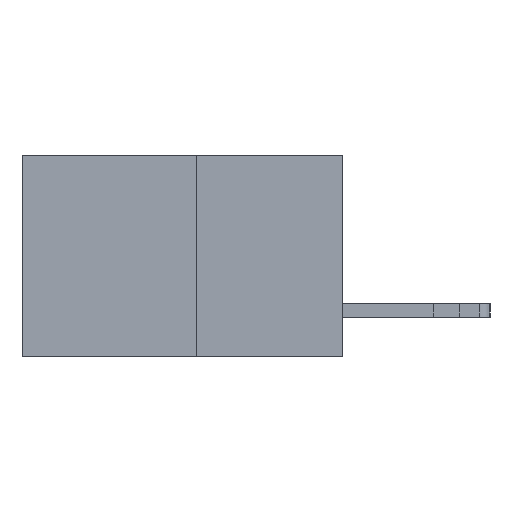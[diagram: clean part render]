
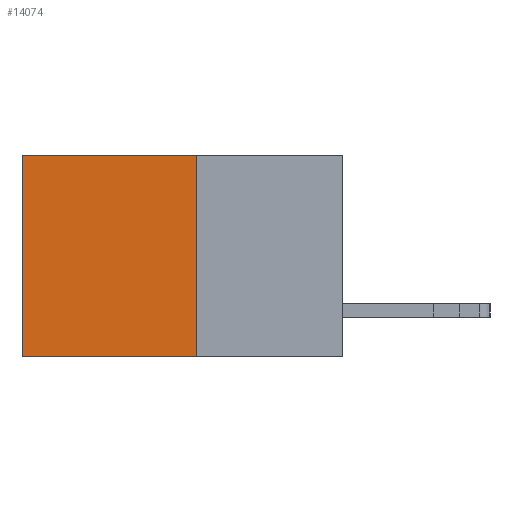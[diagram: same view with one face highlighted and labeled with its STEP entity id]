
A CAD part, left-side view. The second image highlights one B-rep face of the part: STEP entity #14074.
In plain terms, the highlighted planar face has unit normal (-1, 0, 0).
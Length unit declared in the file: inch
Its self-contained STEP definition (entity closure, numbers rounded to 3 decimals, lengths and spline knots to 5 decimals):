
#110 = CARTESIAN_POINT ( 'NONE',  ( 0.277, 0.27, -0.37 ) ) ;
#305 = EDGE_CURVE ( 'NONE', #2787, #11590, #13368, .T. ) ;
#1019 = DIRECTION ( 'NONE',  ( 0., 1., 0. ) ) ;
#1151 = EDGE_CURVE ( 'NONE', #8739, #3783, #10831, .T. ) ;
#1374 = CARTESIAN_POINT ( 'NONE',  ( 0.277, 0.59, 0. ) ) ;
#2718 = PLANE ( 'NONE',  #10328 ) ;
#2787 = VERTEX_POINT ( 'NONE', #14695 ) ;
#3515 = EDGE_CURVE ( 'NONE', #3783, #11590, #11569, .T. ) ;
#3783 = VERTEX_POINT ( 'NONE', #1374 ) ;
#3814 = CARTESIAN_POINT ( 'NONE',  ( 0.277, 0.59, -0.37 ) ) ;
#4017 = DIRECTION ( 'NONE',  ( 0., 0., -1. ) ) ;
#4765 = ORIENTED_EDGE ( 'NONE', *, *, #3515, .T. ) ;
#5447 = CARTESIAN_POINT ( 'NONE',  ( 0.277, 0.27, 0. ) ) ;
#7463 = VECTOR ( 'NONE', #8536, 39.37008 ) ;
#7875 = CARTESIAN_POINT ( 'NONE',  ( 0.277, 0.27, -0.37 ) ) ;
#8052 = DIRECTION ( 'NONE',  ( 0., 0., -1. ) ) ;
#8536 = DIRECTION ( 'NONE',  ( 0., 1., 0. ) ) ;
#8739 = VERTEX_POINT ( 'NONE', #5447 ) ;
#9310 = CARTESIAN_POINT ( 'NONE',  ( 0.277, 0.27, -0.37 ) ) ;
#9673 = VECTOR ( 'NONE', #1019, 39.37008 ) ;
#9764 = ORIENTED_EDGE ( 'NONE', *, *, #1151, .T. ) ;
#10328 = AXIS2_PLACEMENT_3D ( 'NONE', #110, #11689, #4017 ) ;
#10627 = EDGE_CURVE ( 'NONE', #8739, #2787, #12259, .T. ) ;
#10831 = LINE ( 'NONE', #11326, #7463 ) ;
#10972 = FACE_OUTER_BOUND ( 'NONE', #12201, .T. ) ;
#11168 = VECTOR ( 'NONE', #14191, 39.37008 ) ;
#11326 = CARTESIAN_POINT ( 'NONE',  ( 0.277, 0.27, 0. ) ) ;
#11569 = LINE ( 'NONE', #3814, #11168 ) ;
#11590 = VERTEX_POINT ( 'NONE', #16143 ) ;
#11689 = DIRECTION ( 'NONE',  ( 1., 0., 0. ) ) ;
#11889 = VECTOR ( 'NONE', #8052, 39.37008 ) ;
#12201 = EDGE_LOOP ( 'NONE', ( #4765, #15148, #15517, #9764 ) ) ;
#12259 = LINE ( 'NONE', #9310, #11889 ) ;
#13368 = LINE ( 'NONE', #7875, #9673 ) ;
#14074 = ADVANCED_FACE ( 'NONE', ( #10972 ), #2718, .F. ) ;
#14191 = DIRECTION ( 'NONE',  ( 0., 0., -1. ) ) ;
#14695 = CARTESIAN_POINT ( 'NONE',  ( 0.277, 0.27, -0.37 ) ) ;
#15148 = ORIENTED_EDGE ( 'NONE', *, *, #305, .F. ) ;
#15517 = ORIENTED_EDGE ( 'NONE', *, *, #10627, .F. ) ;
#16143 = CARTESIAN_POINT ( 'NONE',  ( 0.277, 0.59, -0.37 ) ) ;
